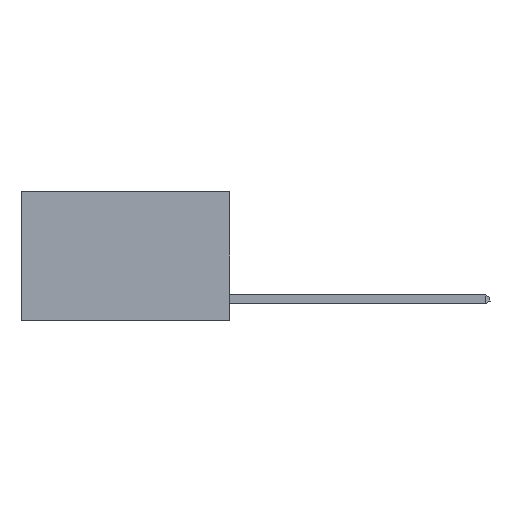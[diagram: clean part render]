
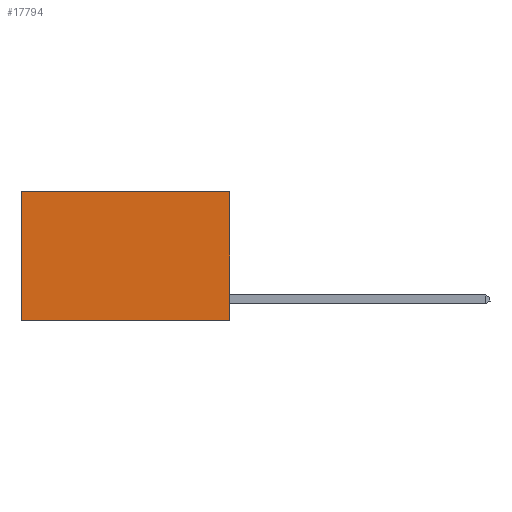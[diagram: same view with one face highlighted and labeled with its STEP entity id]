
A CAD part, left-side view. The second image highlights one B-rep face of the part: STEP entity #17794.
In plain terms, the highlighted planar face has unit normal (-1, 0, 0).
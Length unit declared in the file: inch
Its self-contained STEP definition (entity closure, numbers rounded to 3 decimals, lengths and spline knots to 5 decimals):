
#317 = CARTESIAN_POINT ( 'NONE',  ( 0.2625, 0., 0. ) ) ;
#604 = LINE ( 'NONE', #4549, #12780 ) ;
#742 = CARTESIAN_POINT ( 'NONE',  ( 0.2625, 0., 0. ) ) ;
#1256 = ORIENTED_EDGE ( 'NONE', *, *, #12278, .F. ) ;
#1827 = LINE ( 'NONE', #8355, #17804 ) ;
#2146 = EDGE_CURVE ( 'NONE', #3732, #17273, #13657, .T. ) ;
#2323 = ORIENTED_EDGE ( 'NONE', *, *, #2146, .T. ) ;
#3312 = VERTEX_POINT ( 'NONE', #7337 ) ;
#3552 = DIRECTION ( 'NONE',  ( 0., 0., -1. ) ) ;
#3732 = VERTEX_POINT ( 'NONE', #317 ) ;
#4549 = CARTESIAN_POINT ( 'NONE',  ( 0.2625, 0., 0. ) ) ;
#6332 = PLANE ( 'NONE',  #12154 ) ;
#7337 = CARTESIAN_POINT ( 'NONE',  ( 0.2625, 0., -0.37 ) ) ;
#8355 = CARTESIAN_POINT ( 'NONE',  ( 0.2625, 0.6, 0. ) ) ;
#8820 = CARTESIAN_POINT ( 'NONE',  ( 0.2625, 0.6, -0.37 ) ) ;
#8873 = EDGE_CURVE ( 'NONE', #3732, #3312, #604, .T. ) ;
#8960 = DIRECTION ( 'NONE',  ( 0., 1., 0. ) ) ;
#9392 = DIRECTION ( 'NONE',  ( 1., 0., 0. ) ) ;
#10425 = ORIENTED_EDGE ( 'NONE', *, *, #19657, .T. ) ;
#12154 = AXIS2_PLACEMENT_3D ( 'NONE', #16874, #9392, #19748 ) ;
#12278 = EDGE_CURVE ( 'NONE', #3312, #14266, #18372, .T. ) ;
#12780 = VECTOR ( 'NONE', #18241, 39.37008 ) ;
#13657 = LINE ( 'NONE', #742, #17142 ) ;
#14250 = DIRECTION ( 'NONE',  ( 0., 1., 0. ) ) ;
#14266 = VERTEX_POINT ( 'NONE', #8820 ) ;
#15783 = ORIENTED_EDGE ( 'NONE', *, *, #8873, .F. ) ;
#16874 = CARTESIAN_POINT ( 'NONE',  ( 0.2625, 0., 0. ) ) ;
#17085 = CARTESIAN_POINT ( 'NONE',  ( 0.2625, 0.6, 0. ) ) ;
#17142 = VECTOR ( 'NONE', #8960, 39.37008 ) ;
#17156 = CARTESIAN_POINT ( 'NONE',  ( 0.2625, 0., -0.37 ) ) ;
#17273 = VERTEX_POINT ( 'NONE', #17085 ) ;
#17794 = ADVANCED_FACE ( 'NONE', ( #19639 ), #6332, .F. ) ;
#17804 = VECTOR ( 'NONE', #3552, 39.37008 ) ;
#17935 = VECTOR ( 'NONE', #14250, 39.37008 ) ;
#18241 = DIRECTION ( 'NONE',  ( 0., 0., -1. ) ) ;
#18372 = LINE ( 'NONE', #17156, #17935 ) ;
#18750 = EDGE_LOOP ( 'NONE', ( #10425, #1256, #15783, #2323 ) ) ;
#19639 = FACE_OUTER_BOUND ( 'NONE', #18750, .T. ) ;
#19657 = EDGE_CURVE ( 'NONE', #17273, #14266, #1827, .T. ) ;
#19748 = DIRECTION ( 'NONE',  ( 0., 0., -1. ) ) ;
